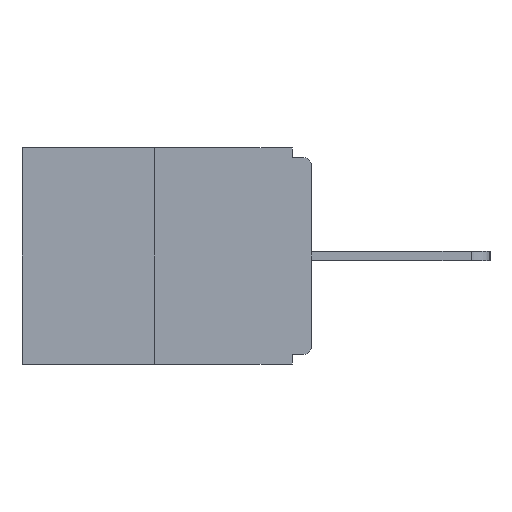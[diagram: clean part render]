
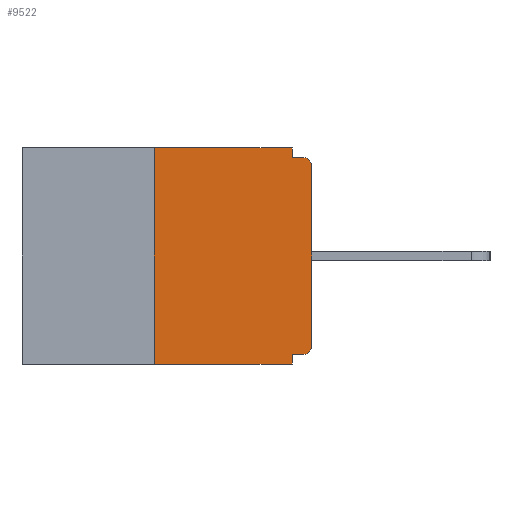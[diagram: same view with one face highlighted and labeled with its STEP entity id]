
A CAD part, left-side view. The second image highlights one B-rep face of the part: STEP entity #9522.
In plain terms, the highlighted planar face has unit normal (-1, 0, 0).
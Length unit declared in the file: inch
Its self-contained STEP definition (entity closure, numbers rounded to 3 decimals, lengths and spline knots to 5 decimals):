
#15 = VERTEX_POINT ( 'NONE', #11954 ) ;
#68 = VERTEX_POINT ( 'NONE', #11326 ) ;
#192 = VERTEX_POINT ( 'NONE', #8119 ) ;
#371 = LINE ( 'NONE', #1438, #8950 ) ;
#508 = VERTEX_POINT ( 'NONE', #3391 ) ;
#749 = CARTESIAN_POINT ( 'NONE',  ( 0., 0.031, -0.328 ) ) ;
#1371 = CARTESIAN_POINT ( 'NONE',  ( 0., 0., -0.03 ) ) ;
#1438 = CARTESIAN_POINT ( 'NONE',  ( 0., 0.25, 0. ) ) ;
#1573 = AXIS2_PLACEMENT_3D ( 'NONE', #5305, #5048, #8776 ) ;
#1697 = VERTEX_POINT ( 'NONE', #749 ) ;
#1720 = EDGE_CURVE ( 'NONE', #6358, #12197, #11122, .T. ) ;
#2151 = EDGE_CURVE ( 'NONE', #1697, #68, #9766, .T. ) ;
#2270 = DIRECTION ( 'NONE',  ( 0., 0., 1. ) ) ;
#2580 = VECTOR ( 'NONE', #10971, 39.37008 ) ;
#2613 = DIRECTION ( 'NONE',  ( 0., -1., 0. ) ) ;
#3169 = VERTEX_POINT ( 'NONE', #1371 ) ;
#3391 = CARTESIAN_POINT ( 'NONE',  ( 0., 0.25, 0. ) ) ;
#3454 = CARTESIAN_POINT ( 'NONE',  ( 0., 0.031, 0. ) ) ;
#3937 = VECTOR ( 'NONE', #12985, 39.37008 ) ;
#4004 = ORIENTED_EDGE ( 'NONE', *, *, #5502, .T. ) ;
#4045 = CARTESIAN_POINT ( 'NONE',  ( 0., 0.031, -0.343 ) ) ;
#4252 = CARTESIAN_POINT ( 'NONE',  ( 0., 0., -0.313 ) ) ;
#4360 = ORIENTED_EDGE ( 'NONE', *, *, #4497, .F. ) ;
#4497 = EDGE_CURVE ( 'NONE', #12197, #10143, #10185, .T. ) ;
#4506 = VECTOR ( 'NONE', #2613, 39.37008 ) ;
#4622 = DIRECTION ( 'NONE',  ( 0., 1., 0. ) ) ;
#4670 = EDGE_CURVE ( 'NONE', #11056, #3169, #5985, .T. ) ;
#4948 = EDGE_CURVE ( 'NONE', #192, #1697, #5791, .T. ) ;
#5048 = DIRECTION ( 'NONE',  ( -1., 0., 0. ) ) ;
#5192 = EDGE_CURVE ( 'NONE', #15, #508, #371, .T. ) ;
#5275 = VECTOR ( 'NONE', #12079, 39.37008 ) ;
#5305 = CARTESIAN_POINT ( 'NONE',  ( 0., 0.015, -0.313 ) ) ;
#5443 = VECTOR ( 'NONE', #4622, 39.37008 ) ;
#5502 = EDGE_CURVE ( 'NONE', #192, #11056, #10161, .T. ) ;
#5590 = AXIS2_PLACEMENT_3D ( 'NONE', #11437, #11419, #11415 ) ;
#5789 = EDGE_LOOP ( 'NONE', ( #8895, #11469, #9214, #6643, #12056, #4004, #7004, #12355, #4360, #7364 ) ) ;
#5791 = LINE ( 'NONE', #8726, #5443 ) ;
#5985 = LINE ( 'NONE', #9531, #5275 ) ;
#6242 = DIRECTION ( 'NONE',  ( 0., 0., -1. ) ) ;
#6261 = DIRECTION ( 'NONE',  ( 1., 0., 0. ) ) ;
#6264 = CARTESIAN_POINT ( 'NONE',  ( 0., 0.46, 0. ) ) ;
#6291 = PLANE ( 'NONE',  #13636 ) ;
#6358 = VERTEX_POINT ( 'NONE', #3454 ) ;
#6643 = ORIENTED_EDGE ( 'NONE', *, *, #2151, .F. ) ;
#7004 = ORIENTED_EDGE ( 'NONE', *, *, #4670, .T. ) ;
#7364 = ORIENTED_EDGE ( 'NONE', *, *, #1720, .F. ) ;
#7508 = LINE ( 'NONE', #13041, #4506 ) ;
#7714 = DIRECTION ( 'NONE',  ( 0., -1., 0. ) ) ;
#8119 = CARTESIAN_POINT ( 'NONE',  ( 0., 0.015, -0.328 ) ) ;
#8220 = LINE ( 'NONE', #11634, #13355 ) ;
#8726 = CARTESIAN_POINT ( 'NONE',  ( 0., 0., -0.328 ) ) ;
#8776 = DIRECTION ( 'NONE',  ( 0., 0., -1. ) ) ;
#8799 = EDGE_CURVE ( 'NONE', #508, #6358, #8220, .T. ) ;
#8802 = EDGE_CURVE ( 'NONE', #3169, #10143, #10590, .T. ) ;
#8895 = ORIENTED_EDGE ( 'NONE', *, *, #8799, .F. ) ;
#8950 = VECTOR ( 'NONE', #2270, 39.37008 ) ;
#9214 = ORIENTED_EDGE ( 'NONE', *, *, #11465, .T. ) ;
#9360 = CARTESIAN_POINT ( 'NONE',  ( 0., 0., -0.015 ) ) ;
#9522 = ADVANCED_FACE ( 'NONE', ( #11752 ), #6291, .F. ) ;
#9531 = CARTESIAN_POINT ( 'NONE',  ( 0., 0., 0. ) ) ;
#9766 = LINE ( 'NONE', #4045, #3937 ) ;
#9893 = VECTOR ( 'NONE', #7714, 39.37008 ) ;
#10143 = VERTEX_POINT ( 'NONE', #10567 ) ;
#10161 = CIRCLE ( 'NONE', #1573, 0.015 ) ;
#10185 = LINE ( 'NONE', #9360, #9893 ) ;
#10567 = CARTESIAN_POINT ( 'NONE',  ( 0., 0.015, -0.015 ) ) ;
#10590 = CIRCLE ( 'NONE', #5590, 0.015 ) ;
#10971 = DIRECTION ( 'NONE',  ( 0., 0., -1. ) ) ;
#11056 = VERTEX_POINT ( 'NONE', #4252 ) ;
#11122 = LINE ( 'NONE', #11207, #2580 ) ;
#11192 = CARTESIAN_POINT ( 'NONE',  ( 0., 0.031, -0.015 ) ) ;
#11207 = CARTESIAN_POINT ( 'NONE',  ( 0., 0.031, 0. ) ) ;
#11326 = CARTESIAN_POINT ( 'NONE',  ( 0., 0.031, -0.343 ) ) ;
#11415 = DIRECTION ( 'NONE',  ( 0., 0., -1. ) ) ;
#11419 = DIRECTION ( 'NONE',  ( -1., 0., 0. ) ) ;
#11437 = CARTESIAN_POINT ( 'NONE',  ( 0., 0.015, -0.03 ) ) ;
#11465 = EDGE_CURVE ( 'NONE', #15, #68, #7508, .T. ) ;
#11469 = ORIENTED_EDGE ( 'NONE', *, *, #5192, .F. ) ;
#11634 = CARTESIAN_POINT ( 'NONE',  ( 0., 0.46, 0. ) ) ;
#11657 = DIRECTION ( 'NONE',  ( 0., -1., 0. ) ) ;
#11752 = FACE_OUTER_BOUND ( 'NONE', #5789, .T. ) ;
#11954 = CARTESIAN_POINT ( 'NONE',  ( 0., 0.25, -0.343 ) ) ;
#12056 = ORIENTED_EDGE ( 'NONE', *, *, #4948, .F. ) ;
#12079 = DIRECTION ( 'NONE',  ( 0., 0., 1. ) ) ;
#12197 = VERTEX_POINT ( 'NONE', #11192 ) ;
#12355 = ORIENTED_EDGE ( 'NONE', *, *, #8802, .T. ) ;
#12985 = DIRECTION ( 'NONE',  ( 0., 0., -1. ) ) ;
#13041 = CARTESIAN_POINT ( 'NONE',  ( 0., 0.46, -0.343 ) ) ;
#13355 = VECTOR ( 'NONE', #11657, 39.37008 ) ;
#13636 = AXIS2_PLACEMENT_3D ( 'NONE', #6264, #6261, #6242 ) ;
